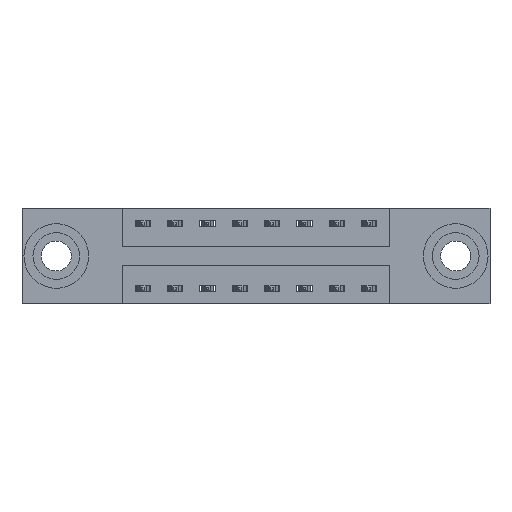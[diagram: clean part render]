
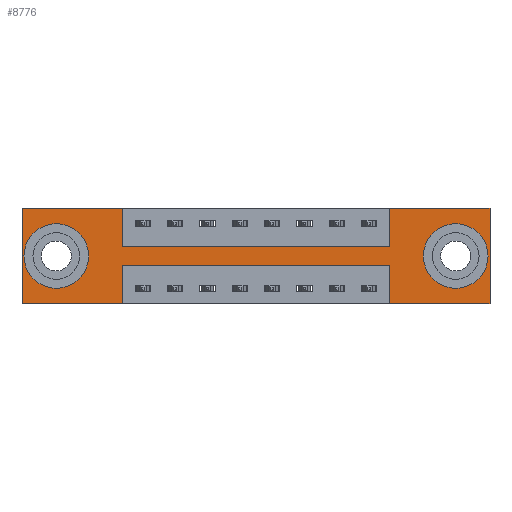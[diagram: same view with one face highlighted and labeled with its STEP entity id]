
A CAD part, front view. The second image highlights one B-rep face of the part: STEP entity #8776.
In plain terms, the highlighted planar face has unit normal (0, -1, 0).
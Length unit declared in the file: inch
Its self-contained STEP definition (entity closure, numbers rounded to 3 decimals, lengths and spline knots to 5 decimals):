
#149 = LINE ( 'NONE', #205, #1112 ) ;
#156 = VECTOR ( 'NONE', #5937, 39.37008 ) ;
#205 = CARTESIAN_POINT ( 'NONE',  ( 0., 0., -0.37 ) ) ;
#213 = VERTEX_POINT ( 'NONE', #6568 ) ;
#224 = DIRECTION ( 'NONE',  ( 0., 0., 1. ) ) ;
#229 = ORIENTED_EDGE ( 'NONE', *, *, #2625, .F. ) ;
#264 = EDGE_LOOP ( 'NONE', ( #5474, #8074 ) ) ;
#314 = LINE ( 'NONE', #7863, #2845 ) ;
#368 = EDGE_CURVE ( 'NONE', #1922, #5306, #2962, .T. ) ;
#409 = CARTESIAN_POINT ( 'NONE',  ( 0., 0., -0.37 ) ) ;
#419 = LINE ( 'NONE', #10469, #4051 ) ;
#428 = EDGE_CURVE ( 'NONE', #5306, #1922, #3320, .T. ) ;
#875 = ORIENTED_EDGE ( 'NONE', *, *, #2596, .F. ) ;
#943 = DIRECTION ( 'NONE',  ( 0., 0., 1. ) ) ;
#1112 = VECTOR ( 'NONE', #6920, 39.37008 ) ;
#1203 = CARTESIAN_POINT ( 'NONE',  ( 1.6775, 0., -0.263 ) ) ;
#1258 = FACE_BOUND ( 'NONE', #264, .T. ) ;
#1430 = DIRECTION ( 'NONE',  ( 0., 0., -1. ) ) ;
#1459 = CARTESIAN_POINT ( 'NONE',  ( 0.3875, 0., -0.15 ) ) ;
#1541 = LINE ( 'NONE', #3456, #5482 ) ;
#1579 = DIRECTION ( 'NONE',  ( 0., 1., 0. ) ) ;
#1754 = AXIS2_PLACEMENT_3D ( 'NONE', #7819, #7765, #224 ) ;
#1759 = LINE ( 'NONE', #1811, #156 ) ;
#1765 = CARTESIAN_POINT ( 'NONE',  ( 0.3875, 0., 0. ) ) ;
#1811 = CARTESIAN_POINT ( 'NONE',  ( 0.3875, 0., -0.37 ) ) ;
#1922 = VERTEX_POINT ( 'NONE', #6450 ) ;
#2114 = LINE ( 'NONE', #5452, #10178 ) ;
#2217 = LINE ( 'NONE', #5397, #10876 ) ;
#2327 = CARTESIAN_POINT ( 'NONE',  ( 1.6775, 0., -0.185 ) ) ;
#2356 = CARTESIAN_POINT ( 'NONE',  ( 1.4225, 0., -0.37 ) ) ;
#2394 = VECTOR ( 'NONE', #3315, 39.37008 ) ;
#2474 = ORIENTED_EDGE ( 'NONE', *, *, #5892, .F. ) ;
#2475 = DIRECTION ( 'NONE',  ( 0., 0., -1. ) ) ;
#2560 = VERTEX_POINT ( 'NONE', #6929 ) ;
#2596 = EDGE_CURVE ( 'NONE', #8554, #10458, #4462, .T. ) ;
#2625 = EDGE_CURVE ( 'NONE', #2669, #7459, #314, .T. ) ;
#2669 = VERTEX_POINT ( 'NONE', #6423 ) ;
#2698 = VECTOR ( 'NONE', #10365, 39.37008 ) ;
#2706 = LINE ( 'NONE', #6063, #3740 ) ;
#2822 = CARTESIAN_POINT ( 'NONE',  ( 0.1325, 0., -0.107 ) ) ;
#2825 = PLANE ( 'NONE',  #9450 ) ;
#2845 = VECTOR ( 'NONE', #3683, 39.37008 ) ;
#2962 = CIRCLE ( 'NONE', #7878, 0.078 ) ;
#3172 = DIRECTION ( 'NONE',  ( 0., 0., 1. ) ) ;
#3315 = DIRECTION ( 'NONE',  ( 1., 0., 0. ) ) ;
#3319 = ORIENTED_EDGE ( 'NONE', *, *, #7188, .F. ) ;
#3320 = CIRCLE ( 'NONE', #1754, 0.078 ) ;
#3402 = VECTOR ( 'NONE', #3172, 39.37008 ) ;
#3456 = CARTESIAN_POINT ( 'NONE',  ( 1.81, 0., 0. ) ) ;
#3465 = ORIENTED_EDGE ( 'NONE', *, *, #3947, .F. ) ;
#3527 = CARTESIAN_POINT ( 'NONE',  ( 0.1325, 0., -0.185 ) ) ;
#3565 = EDGE_LOOP ( 'NONE', ( #8358, #3763 ) ) ;
#3677 = EDGE_CURVE ( 'NONE', #4996, #9267, #7097, .T. ) ;
#3683 = DIRECTION ( 'NONE',  ( 1., 0., 0. ) ) ;
#3694 = ORIENTED_EDGE ( 'NONE', *, *, #10661, .F. ) ;
#3723 = CARTESIAN_POINT ( 'NONE',  ( 1.81, 0., 0. ) ) ;
#3740 = VECTOR ( 'NONE', #4454, 39.37008 ) ;
#3763 = ORIENTED_EDGE ( 'NONE', *, *, #7067, .T. ) ;
#3947 = EDGE_CURVE ( 'NONE', #6160, #4258, #7486, .T. ) ;
#3996 = VERTEX_POINT ( 'NONE', #1203 ) ;
#4051 = VECTOR ( 'NONE', #1430, 39.37008 ) ;
#4258 = VERTEX_POINT ( 'NONE', #1765 ) ;
#4422 = DIRECTION ( 'NONE',  ( 0., 1., 0. ) ) ;
#4454 = DIRECTION ( 'NONE',  ( 1., 0., 0. ) ) ;
#4462 = LINE ( 'NONE', #7807, #2698 ) ;
#4499 = CARTESIAN_POINT ( 'NONE',  ( 0., 0., 0. ) ) ;
#4812 = CARTESIAN_POINT ( 'NONE',  ( 1.6775, 0., -0.185 ) ) ;
#4892 = DIRECTION ( 'NONE',  ( 0., 0., -1. ) ) ;
#4996 = VERTEX_POINT ( 'NONE', #5202 ) ;
#5120 = AXIS2_PLACEMENT_3D ( 'NONE', #2327, #8943, #5676 ) ;
#5168 = CIRCLE ( 'NONE', #8500, 0.078 ) ;
#5202 = CARTESIAN_POINT ( 'NONE',  ( 1.4225, 0., -0.22 ) ) ;
#5306 = VERTEX_POINT ( 'NONE', #2822 ) ;
#5397 = CARTESIAN_POINT ( 'NONE',  ( 0., 0., 0. ) ) ;
#5452 = CARTESIAN_POINT ( 'NONE',  ( 1.4225, 0., -0.37 ) ) ;
#5474 = ORIENTED_EDGE ( 'NONE', *, *, #428, .T. ) ;
#5482 = VECTOR ( 'NONE', #4892, 39.37008 ) ;
#5676 = DIRECTION ( 'NONE',  ( 0., 0., -1. ) ) ;
#5836 = EDGE_CURVE ( 'NONE', #9238, #213, #2706, .T. ) ;
#5844 = EDGE_CURVE ( 'NONE', #2560, #6687, #149, .T. ) ;
#5892 = EDGE_CURVE ( 'NONE', #213, #2669, #9718, .T. ) ;
#5893 = VERTEX_POINT ( 'NONE', #6532 ) ;
#5937 = DIRECTION ( 'NONE',  ( 0., 0., -1. ) ) ;
#6063 = CARTESIAN_POINT ( 'NONE',  ( 0.3875, 0., -0.15 ) ) ;
#6160 = VERTEX_POINT ( 'NONE', #4499 ) ;
#6348 = CIRCLE ( 'NONE', #5120, 0.078 ) ;
#6378 = DIRECTION ( 'NONE',  ( 0., 0., -1. ) ) ;
#6423 = CARTESIAN_POINT ( 'NONE',  ( 1.4225, 0., 0. ) ) ;
#6440 = EDGE_CURVE ( 'NONE', #5893, #3996, #5168, .T. ) ;
#6450 = CARTESIAN_POINT ( 'NONE',  ( 0.1325, 0., -0.263 ) ) ;
#6521 = CARTESIAN_POINT ( 'NONE',  ( 0.3875, 0., -0.22 ) ) ;
#6532 = CARTESIAN_POINT ( 'NONE',  ( 1.6775, 0., -0.107 ) ) ;
#6568 = CARTESIAN_POINT ( 'NONE',  ( 1.4225, 0., -0.15 ) ) ;
#6687 = VERTEX_POINT ( 'NONE', #2356 ) ;
#6920 = DIRECTION ( 'NONE',  ( -1., 0., 0. ) ) ;
#6929 = CARTESIAN_POINT ( 'NONE',  ( 1.81, 0., -0.37 ) ) ;
#6949 = VECTOR ( 'NONE', #7770, 39.37008 ) ;
#6983 = FACE_BOUND ( 'NONE', #3565, .T. ) ;
#7067 = EDGE_CURVE ( 'NONE', #3996, #5893, #6348, .T. ) ;
#7097 = LINE ( 'NONE', #10480, #6949 ) ;
#7188 = EDGE_CURVE ( 'NONE', #7459, #2560, #1541, .T. ) ;
#7196 = ORIENTED_EDGE ( 'NONE', *, *, #5844, .F. ) ;
#7391 = EDGE_CURVE ( 'NONE', #4258, #9238, #419, .T. ) ;
#7459 = VERTEX_POINT ( 'NONE', #3723 ) ;
#7486 = LINE ( 'NONE', #9364, #2394 ) ;
#7698 = ORIENTED_EDGE ( 'NONE', *, *, #3677, .F. ) ;
#7738 = ORIENTED_EDGE ( 'NONE', *, *, #7391, .F. ) ;
#7765 = DIRECTION ( 'NONE',  ( 0., 1., 0. ) ) ;
#7770 = DIRECTION ( 'NONE',  ( -1., 0., 0. ) ) ;
#7807 = CARTESIAN_POINT ( 'NONE',  ( 0., 0., -0.37 ) ) ;
#7819 = CARTESIAN_POINT ( 'NONE',  ( 0.1325, 0., -0.185 ) ) ;
#7863 = CARTESIAN_POINT ( 'NONE',  ( 0., 0., 0. ) ) ;
#7868 = FACE_OUTER_BOUND ( 'NONE', #10537, .T. ) ;
#7878 = AXIS2_PLACEMENT_3D ( 'NONE', #3527, #4422, #943 ) ;
#8074 = ORIENTED_EDGE ( 'NONE', *, *, #368, .T. ) ;
#8149 = CARTESIAN_POINT ( 'NONE',  ( 0.3875, 0., -0.37 ) ) ;
#8358 = ORIENTED_EDGE ( 'NONE', *, *, #6440, .T. ) ;
#8500 = AXIS2_PLACEMENT_3D ( 'NONE', #4812, #1579, #2475 ) ;
#8554 = VERTEX_POINT ( 'NONE', #8149 ) ;
#8712 = EDGE_CURVE ( 'NONE', #10458, #6160, #2217, .T. ) ;
#8776 = ADVANCED_FACE ( 'NONE', ( #6983, #1258, #7868 ), #2825, .T. ) ;
#8799 = DIRECTION ( 'NONE',  ( 0., 0., 1. ) ) ;
#8881 = ORIENTED_EDGE ( 'NONE', *, *, #9987, .F. ) ;
#8943 = DIRECTION ( 'NONE',  ( 0., 1., 0. ) ) ;
#9238 = VERTEX_POINT ( 'NONE', #1459 ) ;
#9267 = VERTEX_POINT ( 'NONE', #6521 ) ;
#9364 = CARTESIAN_POINT ( 'NONE',  ( 0., 0., 0. ) ) ;
#9450 = AXIS2_PLACEMENT_3D ( 'NONE', #9527, #10422, #6378 ) ;
#9527 = CARTESIAN_POINT ( 'NONE',  ( 0., 0., -0.37 ) ) ;
#9718 = LINE ( 'NONE', #9885, #3402 ) ;
#9752 = ORIENTED_EDGE ( 'NONE', *, *, #8712, .F. ) ;
#9885 = CARTESIAN_POINT ( 'NONE',  ( 1.4225, 0., 0. ) ) ;
#9987 = EDGE_CURVE ( 'NONE', #6687, #4996, #2114, .T. ) ;
#10178 = VECTOR ( 'NONE', #8799, 39.37008 ) ;
#10365 = DIRECTION ( 'NONE',  ( -1., 0., 0. ) ) ;
#10369 = DIRECTION ( 'NONE',  ( 0., 0., 1. ) ) ;
#10422 = DIRECTION ( 'NONE',  ( 0., -1., 0. ) ) ;
#10458 = VERTEX_POINT ( 'NONE', #409 ) ;
#10469 = CARTESIAN_POINT ( 'NONE',  ( 0.3875, 0., 0. ) ) ;
#10480 = CARTESIAN_POINT ( 'NONE',  ( 0.3875, 0., -0.22 ) ) ;
#10537 = EDGE_LOOP ( 'NONE', ( #3694, #7698, #8881, #7196, #3319, #229, #2474, #10768, #7738, #3465, #9752, #875 ) ) ;
#10661 = EDGE_CURVE ( 'NONE', #9267, #8554, #1759, .T. ) ;
#10768 = ORIENTED_EDGE ( 'NONE', *, *, #5836, .F. ) ;
#10876 = VECTOR ( 'NONE', #10369, 39.37008 ) ;
